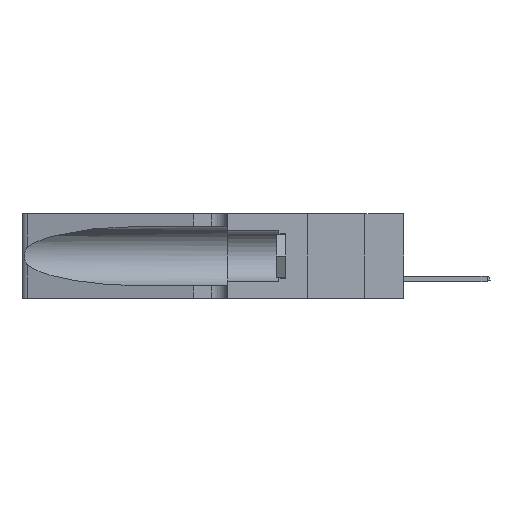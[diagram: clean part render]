
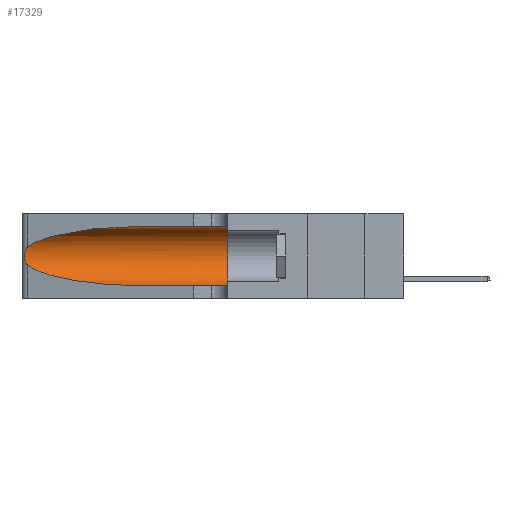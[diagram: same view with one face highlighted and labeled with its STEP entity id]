
A CAD part, left-side view. The second image highlights one B-rep face of the part: STEP entity #17329.
In plain terms, the highlighted cylindrical face has radius 3.308 mm (diameter 6.617 mm), a partial arc.
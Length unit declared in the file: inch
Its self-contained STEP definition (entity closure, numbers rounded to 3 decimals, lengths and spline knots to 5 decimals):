
#296 = CARTESIAN_POINT ( 'NONE',  ( 0.2373, 1.15595, 0.08982 ) ) ;
#323 = CARTESIAN_POINT ( 'NONE',  ( 0.25789, 1.23486, 0.15765 ) ) ;
#382 = CARTESIAN_POINT ( 'NONE',  ( 0.18966, 0.96281, 0.05475 ) ) ;
#397 = CARTESIAN_POINT ( 'NONE',  ( 0.1305, 1.61858, 0.31525 ) ) ;
#1352 = LINE ( 'NONE', #19856, #21294 ) ;
#1821 = CARTESIAN_POINT ( 'NONE',  ( 0.1305, 0.72297, 0.31525 ) ) ;
#2008 = CARTESIAN_POINT ( 'NONE',  ( 0.26075, 1.23896, 0.19203 ) ) ;
#2711 = EDGE_CURVE ( 'NONE', #8758, #4463, #8642, .T. ) ;
#2773 = ORIENTED_EDGE ( 'NONE', *, *, #22165, .F. ) ;
#2998 = DIRECTION ( 'NONE',  ( 0., -1., 0. ) ) ;
#3760 = AXIS2_PLACEMENT_3D ( 'NONE', #15202, #11046, #7434 ) ;
#3860 =( BOUNDED_CURVE ( )  B_SPLINE_CURVE ( 3, ( #1821, #16786, #18856, #18770 ),
 .UNSPECIFIED., .F., .T. ) 
 B_SPLINE_CURVE_WITH_KNOTS ( ( 4, 4 ),
 ( 1.5708, 2.84003 ),
 .UNSPECIFIED. ) 
 CURVE ( )  GEOMETRIC_REPRESENTATION_ITEM ( )  RATIONAL_B_SPLINE_CURVE ( ( 1., 0.87, 0.87, 1. ) ) 
 REPRESENTATION_ITEM ( '' )  );
#4046 = LINE ( 'NONE', #397, #8199 ) ;
#4165 = CARTESIAN_POINT ( 'NONE',  ( 0.25555, 1.22993, 0.14849 ) ) ;
#4463 = VERTEX_POINT ( 'NONE', #19249 ) ;
#4700 = ORIENTED_EDGE ( 'NONE', *, *, #12366, .T. ) ;
#5682 = CARTESIAN_POINT ( 'NONE',  ( 0.25487, 1.22718, 0.14631 ) ) ;
#5962 = EDGE_LOOP ( 'NONE', ( #22736, #4700, #6767, #12134, #8256, #2773 ) ) ;
#6219 = CARTESIAN_POINT ( 'NONE',  ( 0.25639, 1.23186, 0.15144 ) ) ;
#6528 = CARTESIAN_POINT ( 'NONE',  ( 0.25487, 1.22718, 0.22369 ) ) ;
#6755 = CARTESIAN_POINT ( 'NONE',  ( 0.25787, 1.23484, 0.2124 ) ) ;
#6767 = ORIENTED_EDGE ( 'NONE', *, *, #13054, .T. ) ;
#7434 = DIRECTION ( 'NONE',  ( 0., 0., 1. ) ) ;
#7849 = CARTESIAN_POINT ( 'NONE',  ( 0.25639, 1.23184, 0.21858 ) ) ;
#8053 = DIRECTION ( 'NONE',  ( 0., -1., 0. ) ) ;
#8199 = VECTOR ( 'NONE', #8053, 39.37008 ) ;
#8256 = ORIENTED_EDGE ( 'NONE', *, *, #2711, .F. ) ;
#8642 = CIRCLE ( 'NONE', #3760, 0.13025 ) ;
#8758 = VERTEX_POINT ( 'NONE', #19411 ) ;
#9015 = CARTESIAN_POINT ( 'NONE',  ( 0.25555, 1.22994, 0.2215 ) ) ;
#9454 = CYLINDRICAL_SURFACE ( 'NONE', #21507, 0.13025 ) ;
#9794 = CARTESIAN_POINT ( 'NONE',  ( 0.1305, 1.61858, 0.185 ) ) ;
#10106 = VERTEX_POINT ( 'NONE', #16107 ) ;
#10250 =( BOUNDED_CURVE ( )  B_SPLINE_CURVE ( 3, ( #17753, #296, #382, #21427 ),
 .UNSPECIFIED., .F., .F. ) 
 B_SPLINE_CURVE_WITH_KNOTS ( ( 4, 4 ),
 ( 3.44316, 4.71239 ),
 .UNSPECIFIED. ) 
 CURVE ( )  GEOMETRIC_REPRESENTATION_ITEM ( )  RATIONAL_B_SPLINE_CURVE ( ( 1., 0.87, 0.87, 1. ) ) 
 REPRESENTATION_ITEM ( '' )  );
#10926 = FACE_OUTER_BOUND ( 'NONE', #5962, .T. ) ;
#11046 = DIRECTION ( 'NONE',  ( 0., 1., 0. ) ) ;
#11050 = CARTESIAN_POINT ( 'NONE',  ( 0.25487, 1.22718, 0.22369 ) ) ;
#11604 = CARTESIAN_POINT ( 'NONE',  ( 0.26017, 1.23833, 0.17102 ) ) ;
#12134 = ORIENTED_EDGE ( 'NONE', *, *, #22263, .T. ) ;
#12366 = EDGE_CURVE ( 'NONE', #23763, #22466, #19100, .T. ) ;
#13054 = EDGE_CURVE ( 'NONE', #22466, #15948, #10250, .T. ) ;
#13130 = CARTESIAN_POINT ( 'NONE',  ( 0.1305, 0.72297, 0.05475 ) ) ;
#13291 = CARTESIAN_POINT ( 'NONE',  ( 0.26018, 1.23835, 0.19895 ) ) ;
#15202 = CARTESIAN_POINT ( 'NONE',  ( 0.1305, 0.35, 0.185 ) ) ;
#15360 = CARTESIAN_POINT ( 'NONE',  ( 0.26075, 1.23896, 0.178 ) ) ;
#15711 = DIRECTION ( 'NONE',  ( 0., -1., 0. ) ) ;
#15948 = VERTEX_POINT ( 'NONE', #13130 ) ;
#16107 = CARTESIAN_POINT ( 'NONE',  ( 0.1305, 0.72297, 0.31525 ) ) ;
#16786 = CARTESIAN_POINT ( 'NONE',  ( 0.18966, 0.96281, 0.31525 ) ) ;
#17329 = ADVANCED_FACE ( 'NONE', ( #10926 ), #9454, .F. ) ;
#17706 = CARTESIAN_POINT ( 'NONE',  ( 0.25487, 1.22718, 0.14631 ) ) ;
#17753 = CARTESIAN_POINT ( 'NONE',  ( 0.25487, 1.22718, 0.14631 ) ) ;
#18770 = CARTESIAN_POINT ( 'NONE',  ( 0.25487, 1.22718, 0.22369 ) ) ;
#18856 = CARTESIAN_POINT ( 'NONE',  ( 0.2373, 1.15595, 0.28018 ) ) ;
#19100 = B_SPLINE_CURVE_WITH_KNOTS ( 'NONE', 3,
 ( #6528, #9015, #7849, #6755, #24549, #13291, #2008, #15360, #11604, #21296, #323, #6219, #4165, #17706 ),
 .UNSPECIFIED., .F., .F.,
 ( 4, 2, 2, 2, 2, 2, 4 ),
 ( 0., 0.00027, 0.00053, 0.00107, 0.0016, 0.00187, 0.00214 ),
 .UNSPECIFIED. ) ;
#19249 = CARTESIAN_POINT ( 'NONE',  ( 0.1305, 0.35, 0.05475 ) ) ;
#19411 = CARTESIAN_POINT ( 'NONE',  ( 0.1305, 0.35, 0.31525 ) ) ;
#19797 = DIRECTION ( 'NONE',  ( 0., 0., -1. ) ) ;
#19856 = CARTESIAN_POINT ( 'NONE',  ( 0.1305, 1.61858, 0.05475 ) ) ;
#21294 = VECTOR ( 'NONE', #2998, 39.37008 ) ;
#21296 = CARTESIAN_POINT ( 'NONE',  ( 0.25856, 1.23593, 0.16098 ) ) ;
#21427 = CARTESIAN_POINT ( 'NONE',  ( 0.1305, 0.72297, 0.05475 ) ) ;
#21507 = AXIS2_PLACEMENT_3D ( 'NONE', #9794, #15711, #19797 ) ;
#22165 = EDGE_CURVE ( 'NONE', #10106, #8758, #4046, .T. ) ;
#22263 = EDGE_CURVE ( 'NONE', #15948, #4463, #1352, .T. ) ;
#22466 = VERTEX_POINT ( 'NONE', #5682 ) ;
#22736 = ORIENTED_EDGE ( 'NONE', *, *, #24322, .T. ) ;
#23763 = VERTEX_POINT ( 'NONE', #11050 ) ;
#24322 = EDGE_CURVE ( 'NONE', #10106, #23763, #3860, .T. ) ;
#24549 = CARTESIAN_POINT ( 'NONE',  ( 0.25854, 1.2359, 0.20912 ) ) ;
